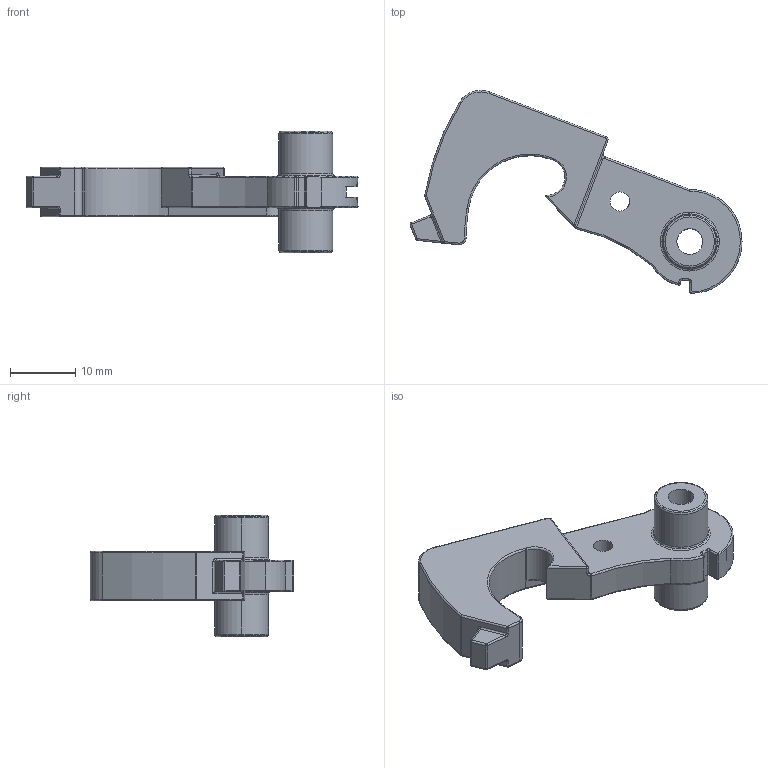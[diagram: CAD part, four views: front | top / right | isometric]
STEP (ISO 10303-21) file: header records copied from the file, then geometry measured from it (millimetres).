
FILE_DESCRIPTION((''),'2;1');
FILE_NAME('M16_HAMMER_V5','2019-01-20T17:52:54',('Cust'),(''),'CREO PARAMETRIC BY PTC INC, 2018300','CREO PARAMETRIC BY PTC INC, 2018300','');
FILE_SCHEMA(('AUTOMOTIVE_DESIGN { 1 0 10303 214 1 1 1 1 }'));
Length unit declared in the file: inch
Products named in the file (1): M16_HAMMER_V5
Bounding box: 50.9 x 31.16 x 18.59 mm (x, y, z)
Volume: 4330 mm3; surface area: 3029.9 mm2
Topology: 1 solids, 1 shells, 162 faces, 480 edges, 315 vertices
Faces by surface type: cylinder 67, torus 42, plane 30, sphere 14, bspline 9
Entity records: 7695 total; most frequent: CARTESIAN_POINT 1754, DIRECTION 1004, ORIENTED_EDGE 946, PRESENTATION_STYLE_ASSIGNMENT 474, STYLED_ITEM 474, CURVE_STYLE 473, EDGE_CURVE 473, AXIS2_PLACEMENT_3D 436
